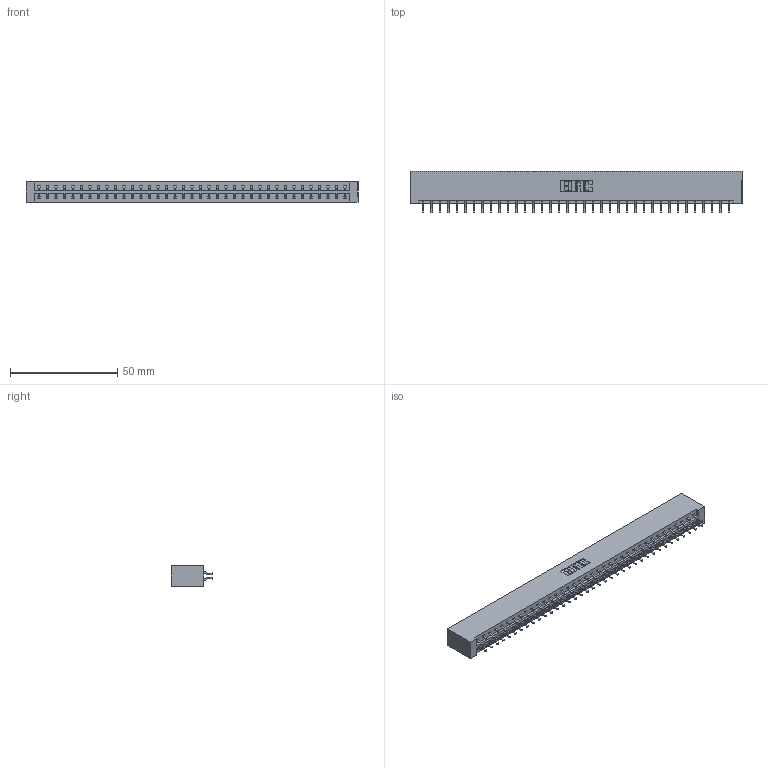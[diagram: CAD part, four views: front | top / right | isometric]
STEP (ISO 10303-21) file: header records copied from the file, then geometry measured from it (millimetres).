
FILE_DESCRIPTION (( 'STEP AP203' ), '1' );
FILE_NAME ('833-074-556-201.STEP', '2020-06-05T17:12:35', ( '' ), ( '' ), 'SwSTEP 2.0', 'SolidWorks 2020', '' );
FILE_SCHEMA (( 'CONFIG_CONTROL_DESIGN' ));
Length unit declared in the file: inch
Products named in the file (3): 833 Part_Lugless; 833-074-556-201; 345-292-001_556 Tail
Assembly tree (75 placements, depth 2):
  833-074-556-201
    833 Part_Lugless
    345-292-001_556 Tail  x74
Bounding box: 154.86 x 19.57 x 9.4 mm (x, y, z)
Volume: 16393.3 mm3; surface area: 19278.5 mm2
Topology: 75 solids, 75 shells, 4398 faces, 13089 edges, 8626 vertices
Faces by surface type: plane 3026, cylinder 1372
Entity records: 24393 total; most frequent: CARTESIAN_POINT 4062, ORIENTED_EDGE 3986, DIRECTION 3461, EDGE_CURVE 1993, VECTOR 1865, LINE 1865, VERTEX_POINT 1326, AXIS2_PLACEMENT_3D 798
